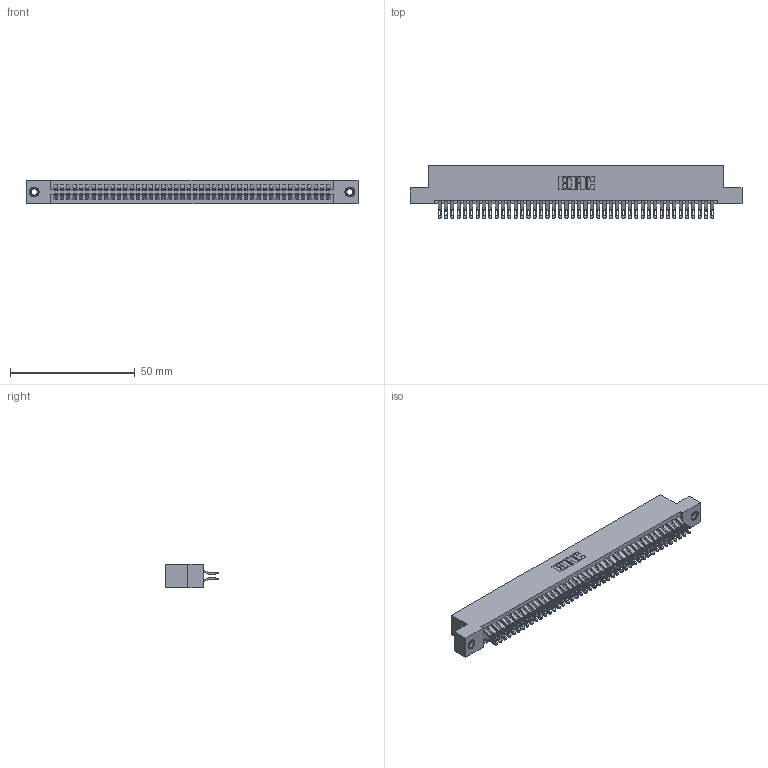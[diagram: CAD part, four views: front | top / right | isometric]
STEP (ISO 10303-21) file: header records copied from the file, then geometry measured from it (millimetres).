
FILE_DESCRIPTION (( 'STEP AP203' ), '1' );
FILE_NAME ('395-088-555-207.STEP', '2018-11-29T00:53:46', ( '' ), ( '' ), 'SwSTEP 2.0', 'SolidWorks 2016', '' );
FILE_SCHEMA (( 'CONFIG_CONTROL_DESIGN' ));
Length unit declared in the file: inch
Products named in the file (4): 345-250-001_345-250-005-103; 345 Part_Flush Mounting Lugs - 0.156 Dia-TI; 345-292-001_555 Tail; 395-088-555-207
Assembly tree (91 placements, depth 2):
  395-088-555-207
    345 Part_Flush Mounting Lugs - 0.156 Dia-TI
    345-292-001_555 Tail  x88
    345-250-001_345-250-005-103  x2
Bounding box: 132.97 x 21.13 x 9.4 mm (x, y, z)
Volume: 13177 mm3; surface area: 20432.3 mm2
Topology: 91 solids, 91 shells, 5114 faces, 16053 edges, 10694 vertices
Faces by surface type: plane 2840, cylinder 2258, cone 12, torus 4
Entity records: 35766 total; most frequent: CARTESIAN_POINT 6009, ORIENTED_EDGE 5906, DIRECTION 5291, EDGE_CURVE 2953, VECTOR 2605, LINE 2605, VERTEX_POINT 1964, AXIS2_PLACEMENT_3D 1343
